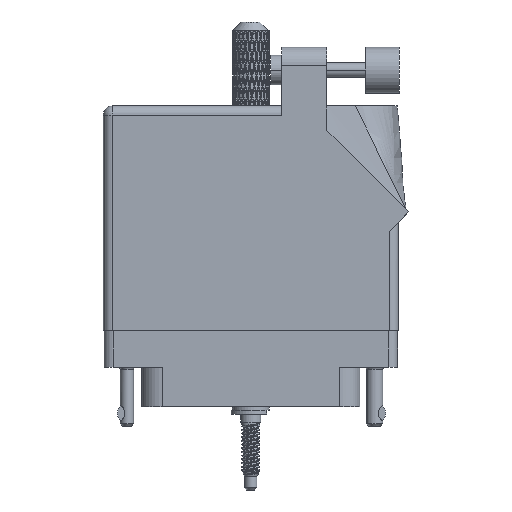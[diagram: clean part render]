
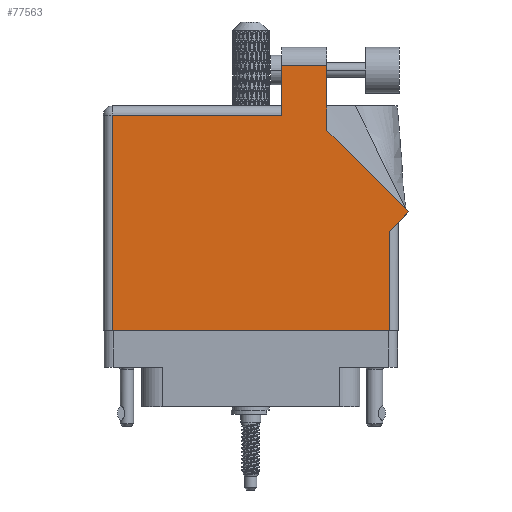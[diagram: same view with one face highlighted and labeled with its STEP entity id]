
A CAD part, front view. The second image highlights one B-rep face of the part: STEP entity #77563.
In plain terms, the highlighted face is planar.
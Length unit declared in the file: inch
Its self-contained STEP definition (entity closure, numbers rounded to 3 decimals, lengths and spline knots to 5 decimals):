
#2058 = ORIENTED_EDGE ( 'NONE', *, *, #112151, .T. ) ;
#7958 = PLANE ( 'NONE',  #85861 ) ;
#9782 = CARTESIAN_POINT ( 'NONE',  ( 0.943, -0.1, 0.455 ) ) ;
#10970 = CARTESIAN_POINT ( 'NONE',  ( 0.212, 1.705, 0.455 ) ) ;
#11238 = EDGE_CURVE ( 'NONE', #87262, #58137, #14184, .T. ) ;
#11728 = LINE ( 'NONE', #17036, #61744 ) ;
#11959 = ORIENTED_EDGE ( 'NONE', *, *, #11238, .T. ) ;
#13842 = LINE ( 'NONE', #69039, #112395 ) ;
#14184 = LINE ( 'NONE', #24637, #55932 ) ;
#14745 = VERTEX_POINT ( 'NONE', #9782 ) ;
#14952 = ORIENTED_EDGE ( 'NONE', *, *, #26831, .T. ) ;
#15826 = DIRECTION ( 'NONE',  ( -1., 0., 0. ) ) ;
#17036 = CARTESIAN_POINT ( 'NONE',  ( 0.943, 0.637, 0.455 ) ) ;
#17300 = DIRECTION ( 'NONE',  ( 0., 1., 0. ) ) ;
#19660 = CARTESIAN_POINT ( 'NONE',  ( 1.005, 0.637, 0.455 ) ) ;
#20535 = DIRECTION ( 'NONE',  ( -0.707, 0.707, 0. ) ) ;
#21869 = DIRECTION ( 'NONE',  ( 0., -1., 0. ) ) ;
#24637 = CARTESIAN_POINT ( 'NONE',  ( 1.07571, 0.70771, 0.455 ) ) ;
#26831 = EDGE_CURVE ( 'NONE', #90341, #77835, #13842, .T. ) ;
#27178 = EDGE_CURVE ( 'NONE', #77835, #31571, #38087, .T. ) ;
#31571 = VERTEX_POINT ( 'NONE', #39467 ) ;
#32081 = DIRECTION ( 'NONE',  ( 0., -1., 0. ) ) ;
#38065 = ORIENTED_EDGE ( 'NONE', *, *, #109567, .T. ) ;
#38087 = LINE ( 'NONE', #68913, #67330 ) ;
#39467 = CARTESIAN_POINT ( 'NONE',  ( -0.943, -0.1, 0.455 ) ) ;
#39850 = CARTESIAN_POINT ( 'NONE',  ( 0.212, 1.43, 0.455 ) ) ;
#41960 = VECTOR ( 'NONE', #17300, 39.37008 ) ;
#43758 = VERTEX_POINT ( 'NONE', #60618 ) ;
#44643 = CARTESIAN_POINT ( 'NONE',  ( -1.005, -0.1, 0.455 ) ) ;
#44666 = DIRECTION ( 'NONE',  ( 0.707, 0.707, 0. ) ) ;
#48471 = CARTESIAN_POINT ( 'NONE',  ( 0.212, 1.368, 0.455 ) ) ;
#51217 = CARTESIAN_POINT ( 'NONE',  ( 0.519, 1.26442, 0.455 ) ) ;
#53733 = VECTOR ( 'NONE', #90654, 39.37008 ) ;
#55932 = VECTOR ( 'NONE', #20535, 39.37008 ) ;
#58137 = VERTEX_POINT ( 'NONE', #63100 ) ;
#58935 = VECTOR ( 'NONE', #21869, 39.37008 ) ;
#60618 = CARTESIAN_POINT ( 'NONE',  ( 0.519, 1.705, 0.455 ) ) ;
#61744 = VECTOR ( 'NONE', #97014, 39.37008 ) ;
#63100 = CARTESIAN_POINT ( 'NONE',  ( 0.519, 1.26442, 0.455 ) ) ;
#63212 = EDGE_CURVE ( 'NONE', #14745, #75842, #11728, .T. ) ;
#63935 = CARTESIAN_POINT ( 'NONE',  ( 0.212, 1.705, 0.455 ) ) ;
#67146 = VECTOR ( 'NONE', #44666, 39.37008 ) ;
#67283 = CARTESIAN_POINT ( 'NONE',  ( -0.943, 1.368, 0.455 ) ) ;
#67330 = VECTOR ( 'NONE', #32081, 39.37008 ) ;
#68913 = CARTESIAN_POINT ( 'NONE',  ( -0.943, -0.1, 0.455 ) ) ;
#69039 = CARTESIAN_POINT ( 'NONE',  ( -1.005, 1.368, 0.455 ) ) ;
#72312 = DIRECTION ( 'NONE',  ( -1., 0., 0. ) ) ;
#73021 = LINE ( 'NONE', #44643, #53733 ) ;
#73959 = CARTESIAN_POINT ( 'NONE',  ( 1.07571, 0.70771, 0.455 ) ) ;
#75842 = VERTEX_POINT ( 'NONE', #77219 ) ;
#77219 = CARTESIAN_POINT ( 'NONE',  ( 0.943, 0.575, 0.455 ) ) ;
#77563 = ADVANCED_FACE ( 'NONE', ( #86382 ), #7958, .F. ) ;
#77835 = VERTEX_POINT ( 'NONE', #67283 ) ;
#80052 = ORIENTED_EDGE ( 'NONE', *, *, #63212, .T. ) ;
#81105 = LINE ( 'NONE', #39850, #58935 ) ;
#83080 = ORIENTED_EDGE ( 'NONE', *, *, #111535, .T. ) ;
#85861 = AXIS2_PLACEMENT_3D ( 'NONE', #105789, #114669, #97222 ) ;
#85913 = VECTOR ( 'NONE', #72312, 39.37008 ) ;
#86382 = FACE_OUTER_BOUND ( 'NONE', #88539, .T. ) ;
#87262 = VERTEX_POINT ( 'NONE', #73959 ) ;
#88539 = EDGE_LOOP ( 'NONE', ( #108280, #104492, #83080, #14952, #112544, #38065, #80052, #2058, #11959 ) ) ;
#89017 = LINE ( 'NONE', #51217, #41960 ) ;
#90341 = VERTEX_POINT ( 'NONE', #48471 ) ;
#90654 = DIRECTION ( 'NONE',  ( 1., 0., 0. ) ) ;
#96304 = LINE ( 'NONE', #19660, #67146 ) ;
#97014 = DIRECTION ( 'NONE',  ( 0., 1., 0. ) ) ;
#97222 = DIRECTION ( 'NONE',  ( -1., 0., 0. ) ) ;
#104492 = ORIENTED_EDGE ( 'NONE', *, *, #107165, .T. ) ;
#105789 = CARTESIAN_POINT ( 'NONE',  ( -1.005, 1.43, 0.455 ) ) ;
#107165 = EDGE_CURVE ( 'NONE', #43758, #112118, #109437, .T. ) ;
#108280 = ORIENTED_EDGE ( 'NONE', *, *, #114259, .T. ) ;
#109437 = LINE ( 'NONE', #10970, #85913 ) ;
#109567 = EDGE_CURVE ( 'NONE', #31571, #14745, #73021, .T. ) ;
#111535 = EDGE_CURVE ( 'NONE', #112118, #90341, #81105, .T. ) ;
#112118 = VERTEX_POINT ( 'NONE', #63935 ) ;
#112151 = EDGE_CURVE ( 'NONE', #75842, #87262, #96304, .T. ) ;
#112395 = VECTOR ( 'NONE', #15826, 39.37008 ) ;
#112544 = ORIENTED_EDGE ( 'NONE', *, *, #27178, .T. ) ;
#114259 = EDGE_CURVE ( 'NONE', #58137, #43758, #89017, .T. ) ;
#114669 = DIRECTION ( 'NONE',  ( 0., 0., -1. ) ) ;
